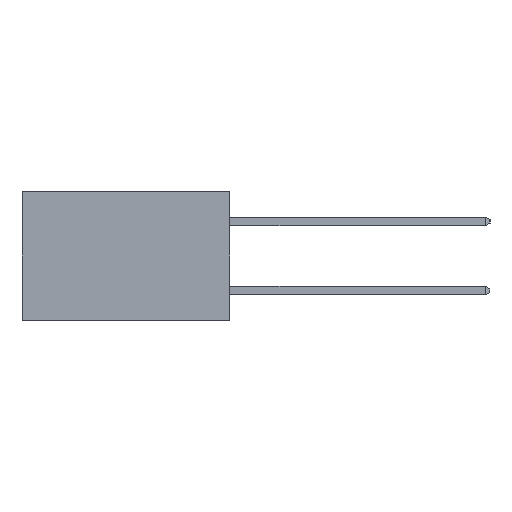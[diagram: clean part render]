
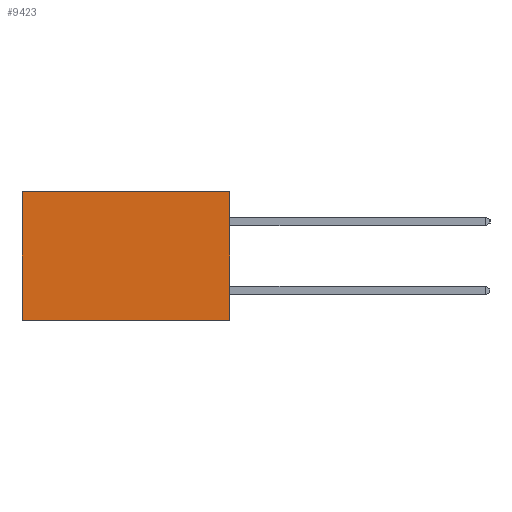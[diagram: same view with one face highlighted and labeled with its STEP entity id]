
A CAD part, left-side view. The second image highlights one B-rep face of the part: STEP entity #9423.
In plain terms, the highlighted planar face has unit normal (-1, 0, 0).
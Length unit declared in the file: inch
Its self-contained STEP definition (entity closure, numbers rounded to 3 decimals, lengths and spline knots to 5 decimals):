
#117 = VECTOR ( 'NONE', #6359, 39.37008 ) ;
#468 = DIRECTION ( 'NONE',  ( 0., 1., 0. ) ) ;
#480 = CARTESIAN_POINT ( 'NONE',  ( 0.298, 0., -0.37 ) ) ;
#599 = CARTESIAN_POINT ( 'NONE',  ( 0.298, 0.6, 0. ) ) ;
#772 = DIRECTION ( 'NONE',  ( 0., 0., -1. ) ) ;
#1252 = CARTESIAN_POINT ( 'NONE',  ( 0.298, 0., -0.37 ) ) ;
#1631 = DIRECTION ( 'NONE',  ( 1., 0., 0. ) ) ;
#2688 = FACE_OUTER_BOUND ( 'NONE', #9044, .T. ) ;
#3572 = CARTESIAN_POINT ( 'NONE',  ( 0.298, 0., 0. ) ) ;
#3577 = LINE ( 'NONE', #599, #5932 ) ;
#3804 = ORIENTED_EDGE ( 'NONE', *, *, #6077, .T. ) ;
#3866 = DIRECTION ( 'NONE',  ( 0., 1., 0. ) ) ;
#4142 = LINE ( 'NONE', #3572, #8890 ) ;
#4613 = VERTEX_POINT ( 'NONE', #9153 ) ;
#5143 = EDGE_CURVE ( 'NONE', #5447, #4613, #10434, .T. ) ;
#5447 = VERTEX_POINT ( 'NONE', #1252 ) ;
#5510 = EDGE_CURVE ( 'NONE', #7562, #9579, #4142, .T. ) ;
#5668 = VECTOR ( 'NONE', #468, 39.37008 ) ;
#5858 = AXIS2_PLACEMENT_3D ( 'NONE', #6032, #1631, #7863 ) ;
#5932 = VECTOR ( 'NONE', #772, 39.37008 ) ;
#6032 = CARTESIAN_POINT ( 'NONE',  ( 0.298, 0., 0. ) ) ;
#6077 = EDGE_CURVE ( 'NONE', #9579, #4613, #3577, .T. ) ;
#6359 = DIRECTION ( 'NONE',  ( 0., 0., -1. ) ) ;
#6512 = CARTESIAN_POINT ( 'NONE',  ( 0.298, 0., 0. ) ) ;
#6517 = ORIENTED_EDGE ( 'NONE', *, *, #5510, .T. ) ;
#7101 = EDGE_CURVE ( 'NONE', #7562, #5447, #9568, .T. ) ;
#7562 = VERTEX_POINT ( 'NONE', #9121 ) ;
#7863 = DIRECTION ( 'NONE',  ( 0., 0., -1. ) ) ;
#8008 = CARTESIAN_POINT ( 'NONE',  ( 0.298, 0.6, 0. ) ) ;
#8065 = ORIENTED_EDGE ( 'NONE', *, *, #5143, .F. ) ;
#8619 = ORIENTED_EDGE ( 'NONE', *, *, #7101, .F. ) ;
#8652 = PLANE ( 'NONE',  #5858 ) ;
#8890 = VECTOR ( 'NONE', #3866, 39.37008 ) ;
#9044 = EDGE_LOOP ( 'NONE', ( #3804, #8065, #8619, #6517 ) ) ;
#9121 = CARTESIAN_POINT ( 'NONE',  ( 0.298, 0., 0. ) ) ;
#9153 = CARTESIAN_POINT ( 'NONE',  ( 0.298, 0.6, -0.37 ) ) ;
#9423 = ADVANCED_FACE ( 'NONE', ( #2688 ), #8652, .F. ) ;
#9568 = LINE ( 'NONE', #6512, #117 ) ;
#9579 = VERTEX_POINT ( 'NONE', #8008 ) ;
#10434 = LINE ( 'NONE', #480, #5668 ) ;
